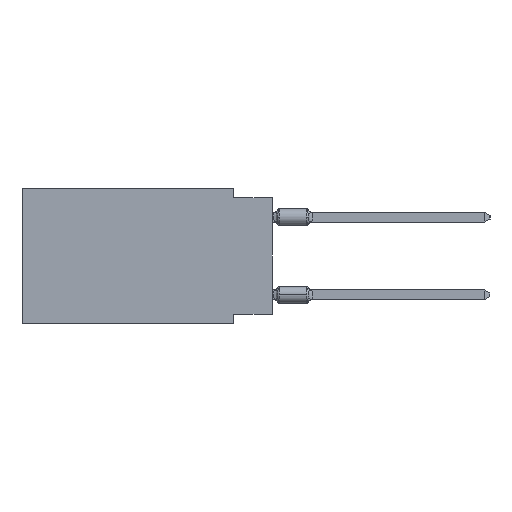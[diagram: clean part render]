
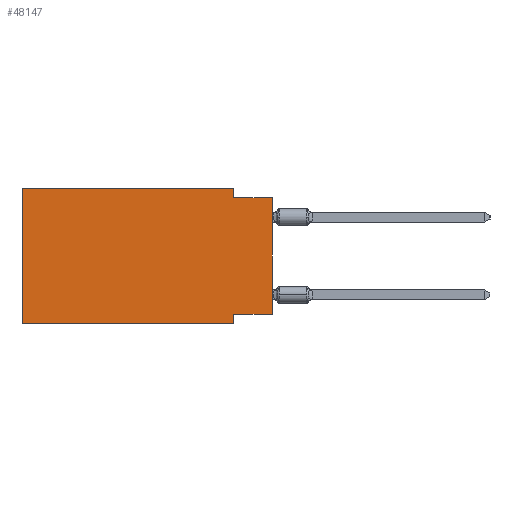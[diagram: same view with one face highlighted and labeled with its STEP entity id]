
A CAD part, left-side view. The second image highlights one B-rep face of the part: STEP entity #48147.
In plain terms, the highlighted planar face has unit normal (-1, 0, 0).
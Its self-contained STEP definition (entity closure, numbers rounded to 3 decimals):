
#1069 = VERTEX_POINT ( 'NONE', #43378 ) ;
#1921 = EDGE_CURVE ( 'NONE', #25523, #45906, #20032, .T. ) ;
#3217 = DIRECTION ( 'NONE',  ( 0., 0., 1. ) ) ;
#3580 = ORIENTED_EDGE ( 'NONE', *, *, #1921, .F. ) ;
#3600 = VECTOR ( 'NONE', #43380, 1000. ) ;
#4066 = DIRECTION ( 'NONE',  ( 0., 0., -1. ) ) ;
#4306 = CARTESIAN_POINT ( 'NONE',  ( 0., 2.54, 0. ) ) ;
#4383 = ORIENTED_EDGE ( 'NONE', *, *, #18808, .F. ) ;
#4872 = DIRECTION ( 'NONE',  ( 0., 0., -1. ) ) ;
#5869 = VECTOR ( 'NONE', #4872, 1000. ) ;
#6347 = VERTEX_POINT ( 'NONE', #9517 ) ;
#6607 = CARTESIAN_POINT ( 'NONE',  ( 0., 2.54, -8.89 ) ) ;
#6770 = LINE ( 'NONE', #37574, #32812 ) ;
#6847 = CARTESIAN_POINT ( 'NONE',  ( 0., 0., 0. ) ) ;
#6919 = EDGE_CURVE ( 'NONE', #22357, #31934, #6770, .T. ) ;
#6923 = LINE ( 'NONE', #44805, #32036 ) ;
#9143 = CARTESIAN_POINT ( 'NONE',  ( 0., 0., -0.635 ) ) ;
#9517 = CARTESIAN_POINT ( 'NONE',  ( 0., 2.54, 0. ) ) ;
#12113 = ORIENTED_EDGE ( 'NONE', *, *, #46941, .F. ) ;
#12139 = EDGE_CURVE ( 'NONE', #22357, #45906, #19234, .T. ) ;
#12169 = DIRECTION ( 'NONE',  ( 0., 0., -1. ) ) ;
#12517 = CARTESIAN_POINT ( 'NONE',  ( 0., 0., -0.635 ) ) ;
#14523 = ORIENTED_EDGE ( 'NONE', *, *, #42587, .F. ) ;
#15967 = DIRECTION ( 'NONE',  ( 0., -1., 0. ) ) ;
#18808 = EDGE_CURVE ( 'NONE', #36268, #19771, #46766, .T. ) ;
#19234 = LINE ( 'NONE', #27553, #28288 ) ;
#19767 = CARTESIAN_POINT ( 'NONE',  ( 0., 16.383, -8.89 ) ) ;
#19771 = VERTEX_POINT ( 'NONE', #12517 ) ;
#20032 = LINE ( 'NONE', #31643, #5869 ) ;
#21236 = ORIENTED_EDGE ( 'NONE', *, *, #43154, .T. ) ;
#22273 = DIRECTION ( 'NONE',  ( 0., 0., 1. ) ) ;
#22357 = VERTEX_POINT ( 'NONE', #19767 ) ;
#24293 = ORIENTED_EDGE ( 'NONE', *, *, #46417, .F. ) ;
#24445 = CARTESIAN_POINT ( 'NONE',  ( 0., 16.383, 0. ) ) ;
#25523 = VERTEX_POINT ( 'NONE', #33544 ) ;
#25628 = VECTOR ( 'NONE', #15967, 1000. ) ;
#25892 = DIRECTION ( 'NONE',  ( 0., 1., 0. ) ) ;
#27313 = LINE ( 'NONE', #4306, #37393 ) ;
#27323 = PLANE ( 'NONE',  #47134 ) ;
#27553 = CARTESIAN_POINT ( 'NONE',  ( 0., 16.383, -8.89 ) ) ;
#27682 = ORIENTED_EDGE ( 'NONE', *, *, #6919, .F. ) ;
#28288 = VECTOR ( 'NONE', #42950, 1000. ) ;
#29300 = ORIENTED_EDGE ( 'NONE', *, *, #12139, .T. ) ;
#29349 = VECTOR ( 'NONE', #22273, 1000. ) ;
#29834 = LINE ( 'NONE', #6847, #29349 ) ;
#31643 = CARTESIAN_POINT ( 'NONE',  ( 0., 2.54, -8.89 ) ) ;
#31934 = VERTEX_POINT ( 'NONE', #32966 ) ;
#32036 = VECTOR ( 'NONE', #25892, 1000. ) ;
#32750 = LINE ( 'NONE', #24445, #3600 ) ;
#32812 = VECTOR ( 'NONE', #3217, 1000. ) ;
#32966 = CARTESIAN_POINT ( 'NONE',  ( 0., 16.383, 0. ) ) ;
#33544 = CARTESIAN_POINT ( 'NONE',  ( 0., 2.54, -8.255 ) ) ;
#36268 = VERTEX_POINT ( 'NONE', #45918 ) ;
#37393 = VECTOR ( 'NONE', #4066, 1000. ) ;
#37574 = CARTESIAN_POINT ( 'NONE',  ( 0., 16.383, 0. ) ) ;
#39184 = FACE_OUTER_BOUND ( 'NONE', #42030, .T. ) ;
#42030 = EDGE_LOOP ( 'NONE', ( #21236, #4383, #12113, #14523, #27682, #29300, #3580, #24293 ) ) ;
#42472 = CARTESIAN_POINT ( 'NONE',  ( 0., 16.383, 0. ) ) ;
#42587 = EDGE_CURVE ( 'NONE', #31934, #6347, #32750, .T. ) ;
#42724 = DIRECTION ( 'NONE',  ( 1., 0., 0. ) ) ;
#42950 = DIRECTION ( 'NONE',  ( 0., -1., 0. ) ) ;
#43154 = EDGE_CURVE ( 'NONE', #1069, #19771, #29834, .T. ) ;
#43378 = CARTESIAN_POINT ( 'NONE',  ( 0., 0., -8.255 ) ) ;
#43380 = DIRECTION ( 'NONE',  ( 0., -1., 0. ) ) ;
#44805 = CARTESIAN_POINT ( 'NONE',  ( 0., 0., -8.255 ) ) ;
#45906 = VERTEX_POINT ( 'NONE', #6607 ) ;
#45918 = CARTESIAN_POINT ( 'NONE',  ( 0., 2.54, -0.635 ) ) ;
#46417 = EDGE_CURVE ( 'NONE', #1069, #25523, #6923, .T. ) ;
#46766 = LINE ( 'NONE', #9143, #25628 ) ;
#46941 = EDGE_CURVE ( 'NONE', #6347, #36268, #27313, .T. ) ;
#47134 = AXIS2_PLACEMENT_3D ( 'NONE', #42472, #42724, #12169 ) ;
#48147 = ADVANCED_FACE ( 'NONE', ( #39184 ), #27323, .F. ) ;
